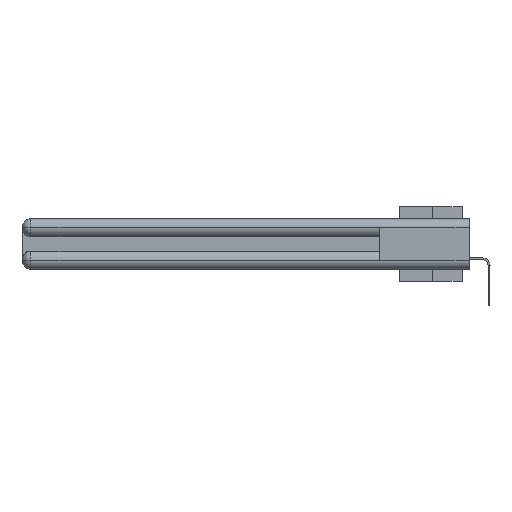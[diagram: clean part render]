
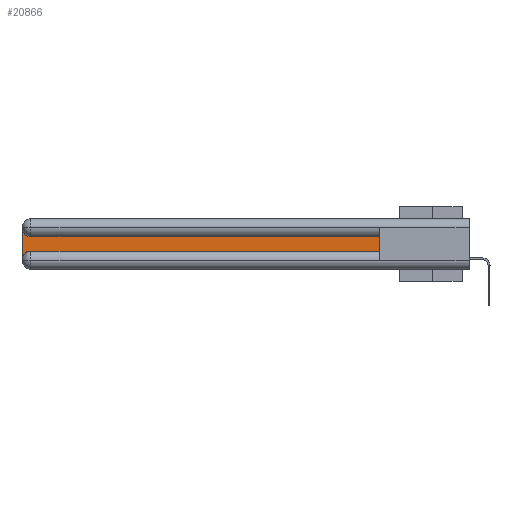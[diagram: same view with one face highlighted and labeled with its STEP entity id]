
A CAD part, left-side view. The second image highlights one B-rep face of the part: STEP entity #20866.
In plain terms, the highlighted planar face has unit normal (-1, 0, 0).
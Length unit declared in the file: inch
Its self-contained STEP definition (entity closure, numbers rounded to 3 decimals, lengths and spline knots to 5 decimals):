
#74 = DIRECTION ( 'NONE',  ( 0., -1., 0. ) ) ;
#289 = LINE ( 'NONE', #2683, #29526 ) ;
#425 = ORIENTED_EDGE ( 'NONE', *, *, #16220, .T. ) ;
#1289 = EDGE_CURVE ( 'NONE', #33480, #8702, #27593, .T. ) ;
#1292 = AXIS2_PLACEMENT_3D ( 'NONE', #20387, #4601, #20064 ) ;
#2683 = CARTESIAN_POINT ( 'NONE',  ( 0.075, 0.6, -0.2175 ) ) ;
#3115 = LINE ( 'NONE', #4371, #8374 ) ;
#3198 = LINE ( 'NONE', #24584, #28754 ) ;
#4037 = DIRECTION ( 'NONE',  ( 0., 0., 1. ) ) ;
#4144 = VERTEX_POINT ( 'NONE', #24727 ) ;
#4371 = CARTESIAN_POINT ( 'NONE',  ( 0.075, 0.6, -0.1225 ) ) ;
#4549 = FACE_OUTER_BOUND ( 'NONE', #4862, .T. ) ;
#4587 = DIRECTION ( 'NONE',  ( 0., 1., 0. ) ) ;
#4601 = DIRECTION ( 'NONE',  ( 1., 0., 0. ) ) ;
#4862 = EDGE_LOOP ( 'NONE', ( #8217, #27793, #26530, #425, #28385, #20518 ) ) ;
#5504 = VERTEX_POINT ( 'NONE', #8002 ) ;
#6847 = AXIS2_PLACEMENT_3D ( 'NONE', #21524, #13566, #21416 ) ;
#7051 = CARTESIAN_POINT ( 'NONE',  ( 0.075, 2.94, -0.1225 ) ) ;
#7687 = VECTOR ( 'NONE', #31079, 39.37008 ) ;
#8002 = CARTESIAN_POINT ( 'NONE',  ( 0.075, 2.94, -0.2175 ) ) ;
#8217 = ORIENTED_EDGE ( 'NONE', *, *, #28848, .T. ) ;
#8374 = VECTOR ( 'NONE', #4587, 39.37008 ) ;
#8702 = VERTEX_POINT ( 'NONE', #16724 ) ;
#13566 = DIRECTION ( 'NONE',  ( 1., 0., 0. ) ) ;
#16099 = CIRCLE ( 'NONE', #19937, 0.06 ) ;
#16220 = EDGE_CURVE ( 'NONE', #8702, #5504, #33310, .T. ) ;
#16724 = CARTESIAN_POINT ( 'NONE',  ( 0.075, 3., -0.2775 ) ) ;
#17015 = VERTEX_POINT ( 'NONE', #7051 ) ;
#17987 = DIRECTION ( 'NONE',  ( 0., 0., -1. ) ) ;
#18473 = EDGE_CURVE ( 'NONE', #17015, #33480, #16099, .T. ) ;
#19937 = AXIS2_PLACEMENT_3D ( 'NONE', #30894, #33516, #17987 ) ;
#20064 = DIRECTION ( 'NONE',  ( 0., 0., -1. ) ) ;
#20278 = PLANE ( 'NONE',  #1292 ) ;
#20387 = CARTESIAN_POINT ( 'NONE',  ( 0.075, 3., -0.1225 ) ) ;
#20518 = ORIENTED_EDGE ( 'NONE', *, *, #30386, .T. ) ;
#20866 = ADVANCED_FACE ( 'NONE', ( #4549 ), #20278, .F. ) ;
#21416 = DIRECTION ( 'NONE',  ( 0., 0., -1. ) ) ;
#21480 = CARTESIAN_POINT ( 'NONE',  ( 0.075, 0.6, -0.1225 ) ) ;
#21524 = CARTESIAN_POINT ( 'NONE',  ( 0.075, 2.94, -0.2775 ) ) ;
#23670 = EDGE_CURVE ( 'NONE', #5504, #4144, #289, .T. ) ;
#24584 = CARTESIAN_POINT ( 'NONE',  ( 0.075, 0.6, -0.2175 ) ) ;
#24727 = CARTESIAN_POINT ( 'NONE',  ( 0.075, 0.6, -0.2175 ) ) ;
#26530 = ORIENTED_EDGE ( 'NONE', *, *, #1289, .T. ) ;
#27593 = LINE ( 'NONE', #30845, #7687 ) ;
#27793 = ORIENTED_EDGE ( 'NONE', *, *, #18473, .T. ) ;
#28385 = ORIENTED_EDGE ( 'NONE', *, *, #23670, .T. ) ;
#28754 = VECTOR ( 'NONE', #4037, 39.37008 ) ;
#28848 = EDGE_CURVE ( 'NONE', #31953, #17015, #3115, .T. ) ;
#29526 = VECTOR ( 'NONE', #74, 39.37008 ) ;
#30386 = EDGE_CURVE ( 'NONE', #4144, #31953, #3198, .T. ) ;
#30777 = CARTESIAN_POINT ( 'NONE',  ( 0.075, 3., -0.0625 ) ) ;
#30845 = CARTESIAN_POINT ( 'NONE',  ( 0.075, 3., -0.2175 ) ) ;
#30894 = CARTESIAN_POINT ( 'NONE',  ( 0.075, 2.94, -0.0625 ) ) ;
#31079 = DIRECTION ( 'NONE',  ( 0., 0., -1. ) ) ;
#31953 = VERTEX_POINT ( 'NONE', #21480 ) ;
#33310 = CIRCLE ( 'NONE', #6847, 0.06 ) ;
#33480 = VERTEX_POINT ( 'NONE', #30777 ) ;
#33516 = DIRECTION ( 'NONE',  ( 1., 0., 0. ) ) ;
